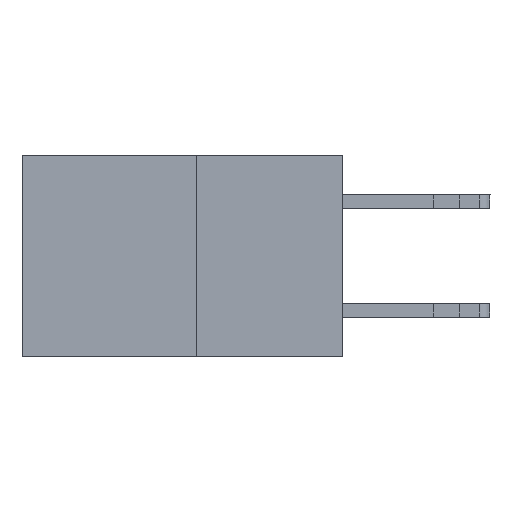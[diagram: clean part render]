
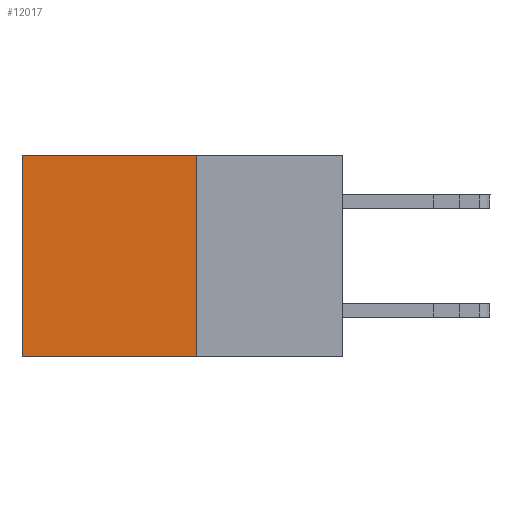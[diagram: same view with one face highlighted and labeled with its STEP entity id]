
A CAD part, left-side view. The second image highlights one B-rep face of the part: STEP entity #12017.
In plain terms, the highlighted planar face has unit normal (-1, 0, 0).
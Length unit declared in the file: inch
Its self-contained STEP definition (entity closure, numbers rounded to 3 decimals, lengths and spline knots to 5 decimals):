
#1497 = FACE_OUTER_BOUND ( 'NONE', #16797, .T. ) ;
#1575 = ORIENTED_EDGE ( 'NONE', *, *, #26163, .F. ) ;
#1941 = CARTESIAN_POINT ( 'NONE',  ( 0.277, 0.59, -0.37 ) ) ;
#2116 = VERTEX_POINT ( 'NONE', #13289 ) ;
#3454 = CARTESIAN_POINT ( 'NONE',  ( 0.277, 0.27, 0. ) ) ;
#3803 = VECTOR ( 'NONE', #14766, 39.37008 ) ;
#3858 = CARTESIAN_POINT ( 'NONE',  ( 0.277, 0.27, -0.37 ) ) ;
#4475 = CARTESIAN_POINT ( 'NONE',  ( 0.277, 0.59, 0. ) ) ;
#4789 = LINE ( 'NONE', #1941, #28788 ) ;
#4852 = VERTEX_POINT ( 'NONE', #9346 ) ;
#5759 = LINE ( 'NONE', #29106, #10890 ) ;
#7915 = VERTEX_POINT ( 'NONE', #3454 ) ;
#8576 = DIRECTION ( 'NONE',  ( 1., 0., 0. ) ) ;
#9346 = CARTESIAN_POINT ( 'NONE',  ( 0.277, 0.59, -0.37 ) ) ;
#10578 = CARTESIAN_POINT ( 'NONE',  ( 0.277, 0.27, -0.37 ) ) ;
#10890 = VECTOR ( 'NONE', #16339, 39.37008 ) ;
#11434 = PLANE ( 'NONE',  #18472 ) ;
#11452 = ORIENTED_EDGE ( 'NONE', *, *, #14628, .T. ) ;
#12017 = ADVANCED_FACE ( 'NONE', ( #1497 ), #11434, .F. ) ;
#13289 = CARTESIAN_POINT ( 'NONE',  ( 0.277, 0.27, -0.37 ) ) ;
#13897 = LINE ( 'NONE', #10578, #20883 ) ;
#14628 = EDGE_CURVE ( 'NONE', #24005, #4852, #4789, .T. ) ;
#14766 = DIRECTION ( 'NONE',  ( 0., 1., 0. ) ) ;
#15049 = DIRECTION ( 'NONE',  ( 0., 0., -1. ) ) ;
#16339 = DIRECTION ( 'NONE',  ( 0., 0., -1. ) ) ;
#16797 = EDGE_LOOP ( 'NONE', ( #11452, #1575, #23076, #19329 ) ) ;
#16801 = DIRECTION ( 'NONE',  ( 0., 0., -1. ) ) ;
#18472 = AXIS2_PLACEMENT_3D ( 'NONE', #3858, #8576, #16801 ) ;
#19329 = ORIENTED_EDGE ( 'NONE', *, *, #23458, .T. ) ;
#20883 = VECTOR ( 'NONE', #21151, 39.37008 ) ;
#21151 = DIRECTION ( 'NONE',  ( 0., 1., 0. ) ) ;
#22346 = LINE ( 'NONE', #30058, #3803 ) ;
#23076 = ORIENTED_EDGE ( 'NONE', *, *, #25296, .F. ) ;
#23458 = EDGE_CURVE ( 'NONE', #7915, #24005, #22346, .T. ) ;
#24005 = VERTEX_POINT ( 'NONE', #4475 ) ;
#25296 = EDGE_CURVE ( 'NONE', #7915, #2116, #5759, .T. ) ;
#26163 = EDGE_CURVE ( 'NONE', #2116, #4852, #13897, .T. ) ;
#28788 = VECTOR ( 'NONE', #15049, 39.37008 ) ;
#29106 = CARTESIAN_POINT ( 'NONE',  ( 0.277, 0.27, -0.37 ) ) ;
#30058 = CARTESIAN_POINT ( 'NONE',  ( 0.277, 0.27, 0. ) ) ;
